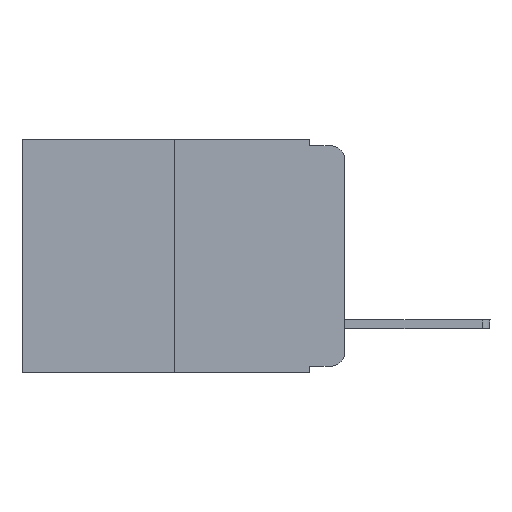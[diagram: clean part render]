
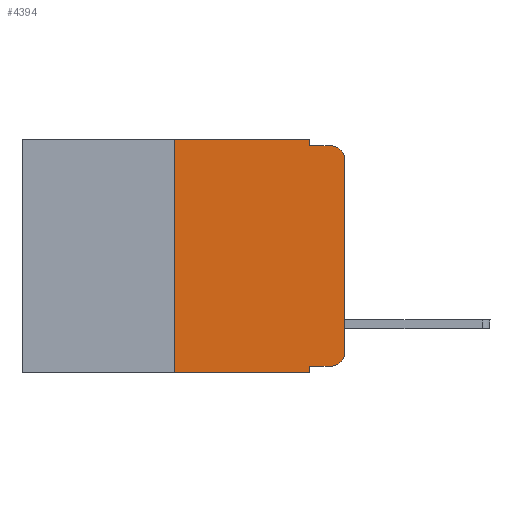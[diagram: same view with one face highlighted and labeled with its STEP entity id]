
A CAD part, left-side view. The second image highlights one B-rep face of the part: STEP entity #4394.
In plain terms, the highlighted planar face has unit normal (-1, 0, 0).
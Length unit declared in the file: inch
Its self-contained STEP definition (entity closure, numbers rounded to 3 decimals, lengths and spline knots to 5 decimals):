
#187 = CARTESIAN_POINT ( 'NONE',  ( 0., 0.25, -0.343 ) ) ;
#268 = LINE ( 'NONE', #4308, #12141 ) ;
#273 = LINE ( 'NONE', #14741, #11808 ) ;
#334 = VERTEX_POINT ( 'NONE', #10250 ) ;
#483 = VECTOR ( 'NONE', #8207, 39.37008 ) ;
#649 = ORIENTED_EDGE ( 'NONE', *, *, #3086, .F. ) ;
#957 = LINE ( 'NONE', #12845, #12691 ) ;
#1101 = ORIENTED_EDGE ( 'NONE', *, *, #4820, .T. ) ;
#1194 = CARTESIAN_POINT ( 'NONE',  ( 0., 0.02, -0.333 ) ) ;
#1343 = DIRECTION ( 'NONE',  ( -1., 0., 0. ) ) ;
#1451 = EDGE_CURVE ( 'NONE', #12984, #16565, #9540, .T. ) ;
#1533 = VERTEX_POINT ( 'NONE', #4469 ) ;
#1608 = EDGE_CURVE ( 'NONE', #3771, #12376, #14995, .T. ) ;
#1951 = CIRCLE ( 'NONE', #7813, 0.02 ) ;
#2261 = VERTEX_POINT ( 'NONE', #10471 ) ;
#2985 = VECTOR ( 'NONE', #14734, 39.37008 ) ;
#3049 = AXIS2_PLACEMENT_3D ( 'NONE', #16385, #8555, #11272 ) ;
#3086 = EDGE_CURVE ( 'NONE', #1533, #10933, #11744, .T. ) ;
#3275 = ORIENTED_EDGE ( 'NONE', *, *, #17012, .F. ) ;
#3631 = ORIENTED_EDGE ( 'NONE', *, *, #1608, .T. ) ;
#3771 = VERTEX_POINT ( 'NONE', #15372 ) ;
#4218 = ORIENTED_EDGE ( 'NONE', *, *, #13036, .T. ) ;
#4308 = CARTESIAN_POINT ( 'NONE',  ( 0., 0.051, -0.333 ) ) ;
#4321 = EDGE_LOOP ( 'NONE', ( #3631, #1101, #649, #13124, #3275, #8135, #15571, #16125, #4218, #12532 ) ) ;
#4331 = CARTESIAN_POINT ( 'NONE',  ( 0., 0.02, -0.01 ) ) ;
#4394 = ADVANCED_FACE ( 'NONE', ( #5201 ), #17094, .F. ) ;
#4469 = CARTESIAN_POINT ( 'NONE',  ( 0., 0.051, -0.01 ) ) ;
#4789 = VECTOR ( 'NONE', #15071, 39.37008 ) ;
#4820 = EDGE_CURVE ( 'NONE', #12376, #10933, #13401, .T. ) ;
#4863 = DIRECTION ( 'NONE',  ( 0., -1., 0. ) ) ;
#5199 = CARTESIAN_POINT ( 'NONE',  ( 0., 0.051, -0.01 ) ) ;
#5201 = FACE_OUTER_BOUND ( 'NONE', #4321, .T. ) ;
#5208 = CARTESIAN_POINT ( 'NONE',  ( 0., 0.02, -0.313 ) ) ;
#5456 = DIRECTION ( 'NONE',  ( 0., -1., 0. ) ) ;
#5558 = EDGE_CURVE ( 'NONE', #10752, #3771, #1951, .T. ) ;
#6507 = CARTESIAN_POINT ( 'NONE',  ( 0., 0.473, 0. ) ) ;
#7458 = LINE ( 'NONE', #12801, #10964 ) ;
#7813 = AXIS2_PLACEMENT_3D ( 'NONE', #5208, #1343, #16320 ) ;
#8135 = ORIENTED_EDGE ( 'NONE', *, *, #1451, .F. ) ;
#8207 = DIRECTION ( 'NONE',  ( 0., -1., 0. ) ) ;
#8555 = DIRECTION ( 'NONE',  ( -1., 0., 0. ) ) ;
#8987 = DIRECTION ( 'NONE',  ( 0., 0., -1. ) ) ;
#9118 = DIRECTION ( 'NONE',  ( 0., 0., -1. ) ) ;
#9383 = CARTESIAN_POINT ( 'NONE',  ( 0., 0.473, -0.343 ) ) ;
#9466 = EDGE_CURVE ( 'NONE', #13685, #334, #273, .T. ) ;
#9540 = LINE ( 'NONE', #10590, #2985 ) ;
#9734 = AXIS2_PLACEMENT_3D ( 'NONE', #6507, #17187, #9118 ) ;
#10250 = CARTESIAN_POINT ( 'NONE',  ( 0., 0.051, -0.343 ) ) ;
#10471 = CARTESIAN_POINT ( 'NONE',  ( 0., 0.051, 0. ) ) ;
#10590 = CARTESIAN_POINT ( 'NONE',  ( 0., 0.25, 0. ) ) ;
#10687 = DIRECTION ( 'NONE',  ( 0., 0., -1. ) ) ;
#10752 = VERTEX_POINT ( 'NONE', #1194 ) ;
#10933 = VERTEX_POINT ( 'NONE', #4331 ) ;
#10964 = VECTOR ( 'NONE', #4863, 39.37008 ) ;
#11029 = CARTESIAN_POINT ( 'NONE',  ( 0., 0., 0. ) ) ;
#11272 = DIRECTION ( 'NONE',  ( 0., 0., -1. ) ) ;
#11520 = EDGE_CURVE ( 'NONE', #2261, #1533, #957, .T. ) ;
#11744 = LINE ( 'NONE', #5199, #483 ) ;
#11808 = VECTOR ( 'NONE', #10687, 39.37008 ) ;
#11818 = VECTOR ( 'NONE', #15558, 39.37008 ) ;
#12141 = VECTOR ( 'NONE', #5456, 39.37008 ) ;
#12376 = VERTEX_POINT ( 'NONE', #15626 ) ;
#12532 = ORIENTED_EDGE ( 'NONE', *, *, #5558, .T. ) ;
#12691 = VECTOR ( 'NONE', #8987, 39.37008 ) ;
#12801 = CARTESIAN_POINT ( 'NONE',  ( 0., 0.473, 0. ) ) ;
#12845 = CARTESIAN_POINT ( 'NONE',  ( 0., 0.051, 0. ) ) ;
#12915 = CARTESIAN_POINT ( 'NONE',  ( 0., 0.25, 0. ) ) ;
#12984 = VERTEX_POINT ( 'NONE', #187 ) ;
#13036 = EDGE_CURVE ( 'NONE', #13685, #10752, #268, .T. ) ;
#13124 = ORIENTED_EDGE ( 'NONE', *, *, #11520, .F. ) ;
#13401 = CIRCLE ( 'NONE', #3049, 0.02 ) ;
#13685 = VERTEX_POINT ( 'NONE', #15905 ) ;
#14734 = DIRECTION ( 'NONE',  ( 0., 0., 1. ) ) ;
#14741 = CARTESIAN_POINT ( 'NONE',  ( 0., 0.051, 0. ) ) ;
#14995 = LINE ( 'NONE', #11029, #4789 ) ;
#15071 = DIRECTION ( 'NONE',  ( 0., 0., 1. ) ) ;
#15372 = CARTESIAN_POINT ( 'NONE',  ( 0., 0., -0.313 ) ) ;
#15407 = EDGE_CURVE ( 'NONE', #12984, #334, #16862, .T. ) ;
#15558 = DIRECTION ( 'NONE',  ( 0., -1., 0. ) ) ;
#15571 = ORIENTED_EDGE ( 'NONE', *, *, #15407, .T. ) ;
#15626 = CARTESIAN_POINT ( 'NONE',  ( 0., 0., -0.03 ) ) ;
#15905 = CARTESIAN_POINT ( 'NONE',  ( 0., 0.051, -0.333 ) ) ;
#16125 = ORIENTED_EDGE ( 'NONE', *, *, #9466, .F. ) ;
#16320 = DIRECTION ( 'NONE',  ( 0., 0., -1. ) ) ;
#16385 = CARTESIAN_POINT ( 'NONE',  ( 0., 0.02, -0.03 ) ) ;
#16565 = VERTEX_POINT ( 'NONE', #12915 ) ;
#16862 = LINE ( 'NONE', #9383, #11818 ) ;
#17012 = EDGE_CURVE ( 'NONE', #16565, #2261, #7458, .T. ) ;
#17094 = PLANE ( 'NONE',  #9734 ) ;
#17187 = DIRECTION ( 'NONE',  ( 1., 0., 0. ) ) ;
